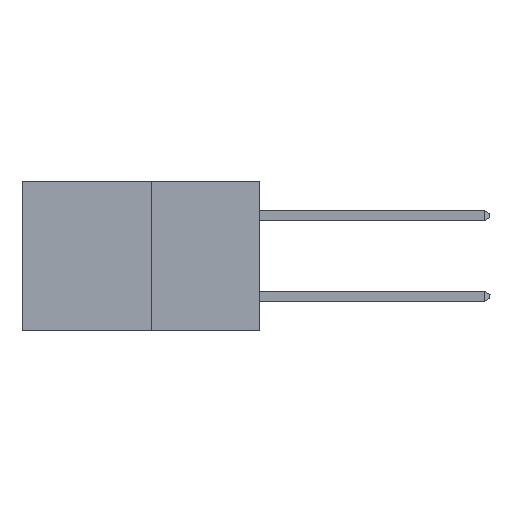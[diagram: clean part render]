
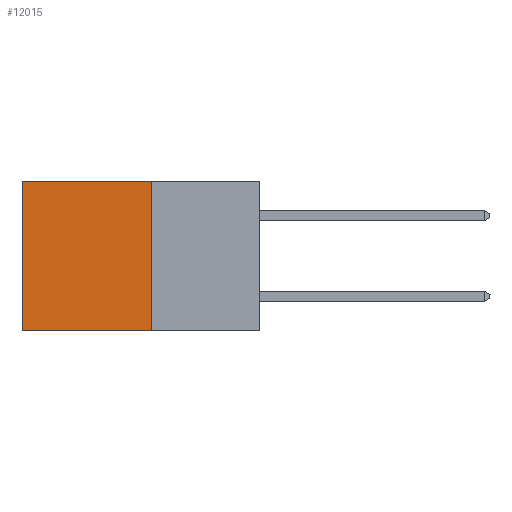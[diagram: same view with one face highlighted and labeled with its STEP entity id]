
A CAD part, left-side view. The second image highlights one B-rep face of the part: STEP entity #12015.
In plain terms, the highlighted planar face has unit normal (-1, 0, 0).
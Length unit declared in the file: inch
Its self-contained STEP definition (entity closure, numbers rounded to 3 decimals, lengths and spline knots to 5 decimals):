
#639 = LINE ( 'NONE', #24611, #26315 ) ;
#1696 = LINE ( 'NONE', #22472, #14300 ) ;
#2229 = ORIENTED_EDGE ( 'NONE', *, *, #6072, .T. ) ;
#2288 = CARTESIAN_POINT ( 'NONE',  ( 0.277, 0.27, 0. ) ) ;
#4595 = DIRECTION ( 'NONE',  ( 0., 0., -1. ) ) ;
#4868 = VECTOR ( 'NONE', #14443, 39.37008 ) ;
#6072 = EDGE_CURVE ( 'NONE', #9542, #19829, #31948, .T. ) ;
#6592 = FACE_OUTER_BOUND ( 'NONE', #10803, .T. ) ;
#6689 = EDGE_CURVE ( 'NONE', #29484, #27368, #1696, .T. ) ;
#7017 = CARTESIAN_POINT ( 'NONE',  ( 0.277, 0.27, -0.37 ) ) ;
#7820 = EDGE_CURVE ( 'NONE', #29484, #9542, #14618, .T. ) ;
#7937 = VECTOR ( 'NONE', #23701, 39.37008 ) ;
#9542 = VERTEX_POINT ( 'NONE', #20480 ) ;
#10803 = EDGE_LOOP ( 'NONE', ( #2229, #27894, #11117, #16498 ) ) ;
#11117 = ORIENTED_EDGE ( 'NONE', *, *, #6689, .F. ) ;
#11988 = CARTESIAN_POINT ( 'NONE',  ( 0.277, 0.27, -0.37 ) ) ;
#12015 = ADVANCED_FACE ( 'NONE', ( #6592 ), #17093, .F. ) ;
#14227 = CARTESIAN_POINT ( 'NONE',  ( 0.277, 0.59, -0.37 ) ) ;
#14300 = VECTOR ( 'NONE', #22444, 39.37008 ) ;
#14443 = DIRECTION ( 'NONE',  ( 0., 0., -1. ) ) ;
#14618 = LINE ( 'NONE', #25496, #7937 ) ;
#16274 = CARTESIAN_POINT ( 'NONE',  ( 0.277, 0.59, -0.37 ) ) ;
#16498 = ORIENTED_EDGE ( 'NONE', *, *, #7820, .T. ) ;
#16928 = AXIS2_PLACEMENT_3D ( 'NONE', #7017, #19595, #4595 ) ;
#17093 = PLANE ( 'NONE',  #16928 ) ;
#19595 = DIRECTION ( 'NONE',  ( 1., 0., 0. ) ) ;
#19829 = VERTEX_POINT ( 'NONE', #16274 ) ;
#20480 = CARTESIAN_POINT ( 'NONE',  ( 0.277, 0.59, 0. ) ) ;
#22444 = DIRECTION ( 'NONE',  ( 0., 0., -1. ) ) ;
#22472 = CARTESIAN_POINT ( 'NONE',  ( 0.277, 0.27, -0.37 ) ) ;
#23701 = DIRECTION ( 'NONE',  ( 0., 1., 0. ) ) ;
#24611 = CARTESIAN_POINT ( 'NONE',  ( 0.277, 0.27, -0.37 ) ) ;
#25496 = CARTESIAN_POINT ( 'NONE',  ( 0.277, 0.27, 0. ) ) ;
#26315 = VECTOR ( 'NONE', #27060, 39.37008 ) ;
#27060 = DIRECTION ( 'NONE',  ( 0., 1., 0. ) ) ;
#27368 = VERTEX_POINT ( 'NONE', #11988 ) ;
#27894 = ORIENTED_EDGE ( 'NONE', *, *, #28757, .F. ) ;
#28757 = EDGE_CURVE ( 'NONE', #27368, #19829, #639, .T. ) ;
#29484 = VERTEX_POINT ( 'NONE', #2288 ) ;
#31948 = LINE ( 'NONE', #14227, #4868 ) ;
